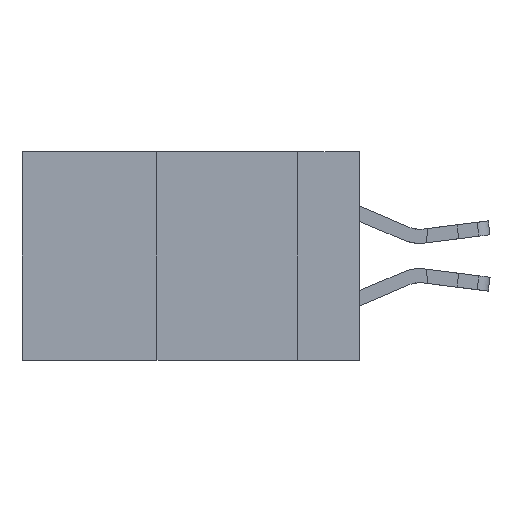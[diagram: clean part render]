
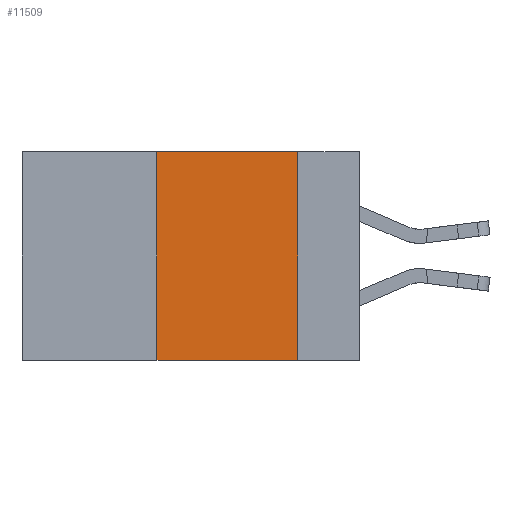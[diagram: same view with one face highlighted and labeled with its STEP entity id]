
A CAD part, left-side view. The second image highlights one B-rep face of the part: STEP entity #11509.
In plain terms, the highlighted planar face has unit normal (-1, 0, 0).
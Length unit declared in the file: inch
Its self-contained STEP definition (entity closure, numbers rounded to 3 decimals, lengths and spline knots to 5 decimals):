
#800 = LINE ( 'NONE', #7532, #13715 ) ;
#946 = CARTESIAN_POINT ( 'NONE',  ( 0., 0.36, 0. ) ) ;
#1750 = VERTEX_POINT ( 'NONE', #16655 ) ;
#2785 = ORIENTED_EDGE ( 'NONE', *, *, #10251, .F. ) ;
#3038 = VECTOR ( 'NONE', #17039, 39.37008 ) ;
#3825 = CARTESIAN_POINT ( 'NONE',  ( 0., 0.6, 0. ) ) ;
#4448 = DIRECTION ( 'NONE',  ( 0., -1., 0. ) ) ;
#7532 = CARTESIAN_POINT ( 'NONE',  ( 0., 0.11, 0. ) ) ;
#9431 = VECTOR ( 'NONE', #28592, 39.37008 ) ;
#10141 = LINE ( 'NONE', #3825, #9431 ) ;
#10251 = EDGE_CURVE ( 'NONE', #1750, #20045, #13759, .T. ) ;
#11024 = CARTESIAN_POINT ( 'NONE',  ( 0., 0.11, 0. ) ) ;
#11183 = EDGE_CURVE ( 'NONE', #26883, #13611, #800, .T. ) ;
#11509 = ADVANCED_FACE ( 'NONE', ( #13686 ), #13741, .F. ) ;
#11627 = DIRECTION ( 'NONE',  ( 1., 0., 0. ) ) ;
#13611 = VERTEX_POINT ( 'NONE', #19752 ) ;
#13686 = FACE_OUTER_BOUND ( 'NONE', #28949, .T. ) ;
#13715 = VECTOR ( 'NONE', #28090, 39.37008 ) ;
#13741 = PLANE ( 'NONE',  #21672 ) ;
#13759 = LINE ( 'NONE', #946, #3038 ) ;
#15355 = CARTESIAN_POINT ( 'NONE',  ( 0., 0.6, 0. ) ) ;
#16386 = LINE ( 'NONE', #20470, #22492 ) ;
#16655 = CARTESIAN_POINT ( 'NONE',  ( 0., 0.36, -0.37 ) ) ;
#17039 = DIRECTION ( 'NONE',  ( 0., 0., 1. ) ) ;
#19148 = EDGE_CURVE ( 'NONE', #20045, #26883, #10141, .T. ) ;
#19752 = CARTESIAN_POINT ( 'NONE',  ( 0., 0.11, -0.37 ) ) ;
#20045 = VERTEX_POINT ( 'NONE', #25165 ) ;
#20236 = ORIENTED_EDGE ( 'NONE', *, *, #22383, .T. ) ;
#20470 = CARTESIAN_POINT ( 'NONE',  ( 0., 0.6, -0.37 ) ) ;
#20775 = ORIENTED_EDGE ( 'NONE', *, *, #19148, .F. ) ;
#21672 = AXIS2_PLACEMENT_3D ( 'NONE', #15355, #11627, #23452 ) ;
#22383 = EDGE_CURVE ( 'NONE', #1750, #13611, #16386, .T. ) ;
#22492 = VECTOR ( 'NONE', #4448, 39.37008 ) ;
#22843 = ORIENTED_EDGE ( 'NONE', *, *, #11183, .F. ) ;
#23452 = DIRECTION ( 'NONE',  ( 0., 0., -1. ) ) ;
#25165 = CARTESIAN_POINT ( 'NONE',  ( 0., 0.36, 0. ) ) ;
#26883 = VERTEX_POINT ( 'NONE', #11024 ) ;
#28090 = DIRECTION ( 'NONE',  ( 0., 0., -1. ) ) ;
#28592 = DIRECTION ( 'NONE',  ( 0., -1., 0. ) ) ;
#28949 = EDGE_LOOP ( 'NONE', ( #22843, #20775, #2785, #20236 ) ) ;
